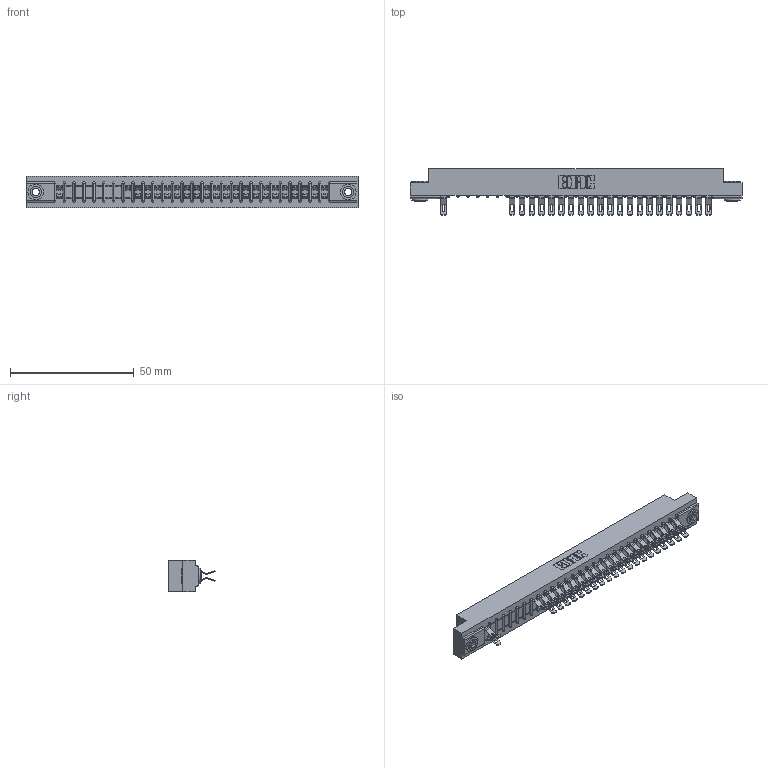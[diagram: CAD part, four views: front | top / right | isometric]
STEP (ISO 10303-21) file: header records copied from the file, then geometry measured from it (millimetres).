
FILE_DESCRIPTION (( 'STEP AP203' ), '1' );
FILE_NAME ('307-056-555-203.STEP', '2018-08-06T06:55:51', ( '' ), ( '' ), 'SwSTEP 2.0', 'SolidWorks 2016', '' );
FILE_SCHEMA (( 'CONFIG_CONTROL_DESIGN' ));
Length unit declared in the file: inch
Products named in the file (4): 307-290-001_555; 345-250-002_345-250-002-102; 307-056-555-203; 307 Part_.156 Dia Mounting Holes
Assembly tree (46 placements, depth 2):
  307-056-555-203
    307 Part_.156 Dia Mounting Holes
    307-290-001_555  x43
    345-250-002_345-250-002-102  x2
Bounding box: 133.96 x 18.75 x 12.7 mm (x, y, z)
Volume: 14106.9 mm3; surface area: 16834.3 mm2
Topology: 46 solids, 46 shells, 2952 faces, 8634 edges, 5616 vertices
Faces by surface type: plane 1634, cylinder 1252, sphere 58, cone 8
Entity records: 27812 total; most frequent: CARTESIAN_POINT 4596, ORIENTED_EDGE 4560, DIRECTION 4516, EDGE_CURVE 2280, VECTOR 1724, LINE 1724, VERTEX_POINT 1476, AXIS2_PLACEMENT_3D 1396
